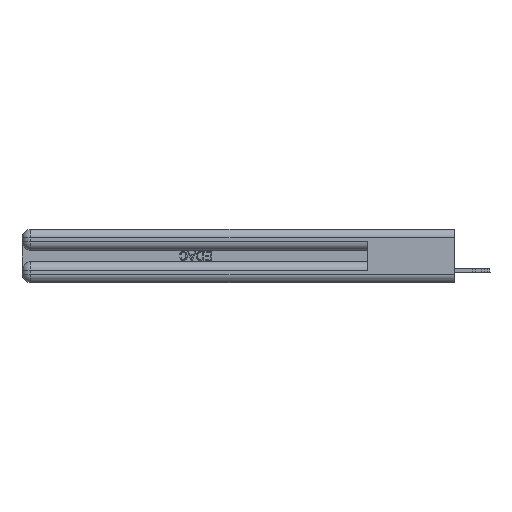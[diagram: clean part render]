
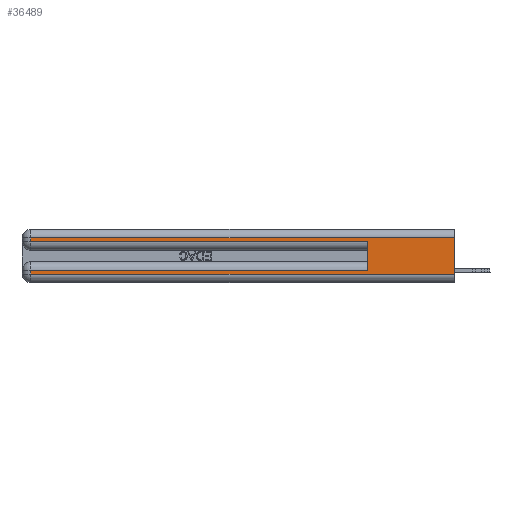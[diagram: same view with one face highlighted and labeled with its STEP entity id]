
A CAD part, left-side view. The second image highlights one B-rep face of the part: STEP entity #36489.
In plain terms, the highlighted planar face has unit normal (-1, 0, 0).
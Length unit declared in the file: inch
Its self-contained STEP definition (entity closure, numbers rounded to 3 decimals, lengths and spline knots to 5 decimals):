
#322 = CARTESIAN_POINT ( 'NONE',  ( 0., 0., 0.37 ) ) ;
#695 = ORIENTED_EDGE ( 'NONE', *, *, #29534, .T. ) ;
#1763 = CARTESIAN_POINT ( 'NONE',  ( 0., 2.94, 0.06 ) ) ;
#2122 = DIRECTION ( 'NONE',  ( 0., 0., -1. ) ) ;
#2434 = ORIENTED_EDGE ( 'NONE', *, *, #5150, .T. ) ;
#2457 = CARTESIAN_POINT ( 'NONE',  ( 0., 0., 0.06 ) ) ;
#2471 = EDGE_CURVE ( 'NONE', #42176, #34559, #11171, .T. ) ;
#3485 = ORIENTED_EDGE ( 'NONE', *, *, #21325, .T. ) ;
#3943 = VECTOR ( 'NONE', #2122, 39.37008 ) ;
#4080 = VECTOR ( 'NONE', #41309, 39.37008 ) ;
#5085 = ORIENTED_EDGE ( 'NONE', *, *, #2471, .T. ) ;
#5150 = EDGE_CURVE ( 'NONE', #10709, #42176, #28893, .T. ) ;
#6854 = CARTESIAN_POINT ( 'NONE',  ( 0., 0., 0.06 ) ) ;
#7877 = LINE ( 'NONE', #22688, #37745 ) ;
#8128 = VECTOR ( 'NONE', #15742, 39.37008 ) ;
#8288 = CARTESIAN_POINT ( 'NONE',  ( 0., 0., 0.31 ) ) ;
#8823 = CARTESIAN_POINT ( 'NONE',  ( 0., 0.6, 0.285 ) ) ;
#8899 = CARTESIAN_POINT ( 'NONE',  ( 0., 2.94, 0.37 ) ) ;
#9119 = DIRECTION ( 'NONE',  ( 0., 0., -1. ) ) ;
#9171 = CARTESIAN_POINT ( 'NONE',  ( 0., 0., 0.31 ) ) ;
#9942 = LINE ( 'NONE', #41065, #35356 ) ;
#10709 = VERTEX_POINT ( 'NONE', #12820 ) ;
#11158 = CARTESIAN_POINT ( 'NONE',  ( 0., 2.94, 0.085 ) ) ;
#11171 = LINE ( 'NONE', #23702, #43117 ) ;
#11332 = VERTEX_POINT ( 'NONE', #11158 ) ;
#12820 = CARTESIAN_POINT ( 'NONE',  ( 0., 2.94, 0.31 ) ) ;
#13073 = CARTESIAN_POINT ( 'NONE',  ( 0., 0., 0.37 ) ) ;
#15742 = DIRECTION ( 'NONE',  ( 0., 1., 0. ) ) ;
#17061 = DIRECTION ( 'NONE',  ( 0., -1., 0. ) ) ;
#18554 = VECTOR ( 'NONE', #17061, 39.37008 ) ;
#19361 = VERTEX_POINT ( 'NONE', #1763 ) ;
#19477 = PLANE ( 'NONE',  #36253 ) ;
#20330 = CARTESIAN_POINT ( 'NONE',  ( 0., 0.6, 0.145 ) ) ;
#21325 = EDGE_CURVE ( 'NONE', #11332, #19361, #9942, .T. ) ;
#22688 = CARTESIAN_POINT ( 'NONE',  ( 0., 0., 0.085 ) ) ;
#23702 = CARTESIAN_POINT ( 'NONE',  ( 0., 0., 0.285 ) ) ;
#24962 = DIRECTION ( 'NONE',  ( 0., 0., -1. ) ) ;
#28893 = LINE ( 'NONE', #8899, #3943 ) ;
#29534 = EDGE_CURVE ( 'NONE', #19361, #32129, #39064, .T. ) ;
#29822 = DIRECTION ( 'NONE',  ( 0., 1., 0. ) ) ;
#30311 = ORIENTED_EDGE ( 'NONE', *, *, #37278, .T. ) ;
#30521 = DIRECTION ( 'NONE',  ( 1., 0., 0. ) ) ;
#30602 = LINE ( 'NONE', #322, #38618 ) ;
#31847 = EDGE_LOOP ( 'NONE', ( #36684, #37469, #2434, #5085, #35416, #30311, #3485, #695 ) ) ;
#32129 = VERTEX_POINT ( 'NONE', #2457 ) ;
#32475 = EDGE_CURVE ( 'NONE', #34235, #32129, #30602, .T. ) ;
#32812 = LINE ( 'NONE', #20330, #4080 ) ;
#34235 = VERTEX_POINT ( 'NONE', #9171 ) ;
#34559 = VERTEX_POINT ( 'NONE', #8823 ) ;
#35112 = VERTEX_POINT ( 'NONE', #43249 ) ;
#35356 = VECTOR ( 'NONE', #37450, 39.37008 ) ;
#35416 = ORIENTED_EDGE ( 'NONE', *, *, #38803, .F. ) ;
#35596 = FACE_OUTER_BOUND ( 'NONE', #31847, .T. ) ;
#36253 = AXIS2_PLACEMENT_3D ( 'NONE', #13073, #30521, #9119 ) ;
#36317 = LINE ( 'NONE', #8288, #8128 ) ;
#36489 = ADVANCED_FACE ( 'NONE', ( #35596 ), #19477, .F. ) ;
#36684 = ORIENTED_EDGE ( 'NONE', *, *, #32475, .F. ) ;
#37278 = EDGE_CURVE ( 'NONE', #35112, #11332, #7877, .T. ) ;
#37450 = DIRECTION ( 'NONE',  ( 0., 0., -1. ) ) ;
#37469 = ORIENTED_EDGE ( 'NONE', *, *, #41791, .T. ) ;
#37745 = VECTOR ( 'NONE', #29822, 39.37008 ) ;
#38618 = VECTOR ( 'NONE', #24962, 39.37008 ) ;
#38803 = EDGE_CURVE ( 'NONE', #35112, #34559, #32812, .T. ) ;
#39064 = LINE ( 'NONE', #6854, #18554 ) ;
#41065 = CARTESIAN_POINT ( 'NONE',  ( 0., 2.94, 0.37 ) ) ;
#41309 = DIRECTION ( 'NONE',  ( 0., 0., 1. ) ) ;
#41791 = EDGE_CURVE ( 'NONE', #34235, #10709, #36317, .T. ) ;
#42176 = VERTEX_POINT ( 'NONE', #42263 ) ;
#42263 = CARTESIAN_POINT ( 'NONE',  ( 0., 2.94, 0.285 ) ) ;
#43117 = VECTOR ( 'NONE', #44223, 39.37008 ) ;
#43249 = CARTESIAN_POINT ( 'NONE',  ( 0., 0.6, 0.085 ) ) ;
#44223 = DIRECTION ( 'NONE',  ( 0., -1., 0. ) ) ;
